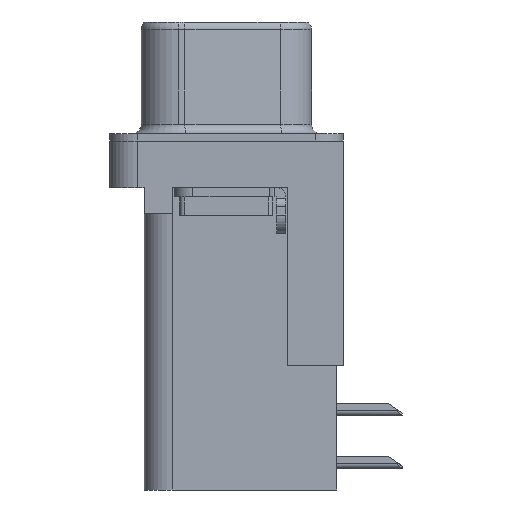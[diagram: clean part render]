
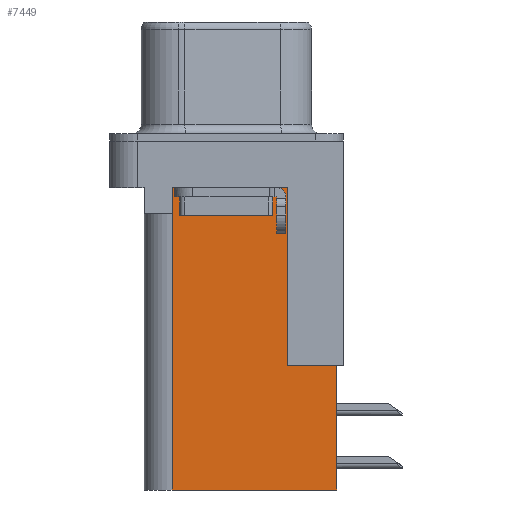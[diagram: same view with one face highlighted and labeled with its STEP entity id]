
A CAD part, left-side view. The second image highlights one B-rep face of the part: STEP entity #7449.
In plain terms, the highlighted planar face has unit normal (-1, 0, 0).
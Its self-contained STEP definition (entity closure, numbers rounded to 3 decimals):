
#61 = EDGE_CURVE ( 'NONE', #4166, #10575, #13281, .T. ) ;
#116 = CARTESIAN_POINT ( 'NONE',  ( 3.79, -3.295, -18.76 ) ) ;
#497 = VECTOR ( 'NONE', #8752, 1000. ) ;
#525 = VERTEX_POINT ( 'NONE', #11522 ) ;
#604 = CARTESIAN_POINT ( 'NONE',  ( 3.79, 2.895, -3.9 ) ) ;
#1216 = ORIENTED_EDGE ( 'NONE', *, *, #10391, .T. ) ;
#1543 = VERTEX_POINT ( 'NONE', #1921 ) ;
#1921 = CARTESIAN_POINT ( 'NONE',  ( 3.79, 2.925, -18.76 ) ) ;
#1950 = ORIENTED_EDGE ( 'NONE', *, *, #4761, .T. ) ;
#2294 = VECTOR ( 'NONE', #6717, 1000. ) ;
#2402 = VECTOR ( 'NONE', #7269, 1000. ) ;
#2490 = VECTOR ( 'NONE', #4081, 1000. ) ;
#2610 = DIRECTION ( 'NONE',  ( 0., 1., 0. ) ) ;
#3317 = VERTEX_POINT ( 'NONE', #9814 ) ;
#3702 = AXIS2_PLACEMENT_3D ( 'NONE', #116, #9983, #2610 ) ;
#4001 = VECTOR ( 'NONE', #10734, 1000. ) ;
#4081 = DIRECTION ( 'NONE',  ( 0., 1., 0. ) ) ;
#4166 = VERTEX_POINT ( 'NONE', #5208 ) ;
#4231 = DIRECTION ( 'NONE',  ( 0., 1., 0. ) ) ;
#4266 = DIRECTION ( 'NONE',  ( 0., 1., 0. ) ) ;
#4658 = EDGE_CURVE ( 'NONE', #9253, #3317, #7698, .T. ) ;
#4761 = EDGE_CURVE ( 'NONE', #3317, #525, #15623, .T. ) ;
#4988 = VERTEX_POINT ( 'NONE', #10867 ) ;
#5208 = CARTESIAN_POINT ( 'NONE',  ( 3.79, -5.925, -12.05 ) ) ;
#5492 = CARTESIAN_POINT ( 'NONE',  ( 3.79, 2.895, -3.9 ) ) ;
#6335 = ORIENTED_EDGE ( 'NONE', *, *, #7844, .T. ) ;
#6582 = VECTOR ( 'NONE', #4266, 1000. ) ;
#6639 = FACE_OUTER_BOUND ( 'NONE', #8283, .T. ) ;
#6717 = DIRECTION ( 'NONE',  ( 0., 0., 1. ) ) ;
#7216 = LINE ( 'NONE', #7931, #9690 ) ;
#7269 = DIRECTION ( 'NONE',  ( 0., 1., 0. ) ) ;
#7449 = ADVANCED_FACE ( 'NONE', ( #6639 ), #8734, .F. ) ;
#7698 = LINE ( 'NONE', #10956, #4001 ) ;
#7844 = EDGE_CURVE ( 'NONE', #12771, #4988, #8922, .T. ) ;
#7931 = CARTESIAN_POINT ( 'NONE',  ( 3.79, -6.295, -12.05 ) ) ;
#8283 = EDGE_LOOP ( 'NONE', ( #1950, #1216, #6335, #9235, #13030, #12469, #13740, #14829 ) ) ;
#8734 = PLANE ( 'NONE',  #3702 ) ;
#8752 = DIRECTION ( 'NONE',  ( 0., 0., -1. ) ) ;
#8922 = LINE ( 'NONE', #15890, #2402 ) ;
#9179 = CARTESIAN_POINT ( 'NONE',  ( 3.79, 2.925, -18.76 ) ) ;
#9183 = CARTESIAN_POINT ( 'NONE',  ( 3.79, -3.295, -18.76 ) ) ;
#9235 = ORIENTED_EDGE ( 'NONE', *, *, #12178, .F. ) ;
#9253 = VERTEX_POINT ( 'NONE', #12428 ) ;
#9469 = LINE ( 'NONE', #604, #12756 ) ;
#9690 = VECTOR ( 'NONE', #4231, 1000. ) ;
#9814 = CARTESIAN_POINT ( 'NONE',  ( 3.79, -3.295, -2.5 ) ) ;
#9853 = LINE ( 'NONE', #9183, #6582 ) ;
#9983 = DIRECTION ( 'NONE',  ( 1., 0., 0. ) ) ;
#10366 = EDGE_CURVE ( 'NONE', #10575, #1543, #9853, .T. ) ;
#10391 = EDGE_CURVE ( 'NONE', #525, #12771, #9469, .T. ) ;
#10575 = VERTEX_POINT ( 'NONE', #10910 ) ;
#10734 = DIRECTION ( 'NONE',  ( 0., 0., 1. ) ) ;
#10847 = CARTESIAN_POINT ( 'NONE',  ( 3.79, -3.295, -2.5 ) ) ;
#10867 = CARTESIAN_POINT ( 'NONE',  ( 3.79, 2.925, -3.9 ) ) ;
#10910 = CARTESIAN_POINT ( 'NONE',  ( 3.79, -5.925, -18.76 ) ) ;
#10956 = CARTESIAN_POINT ( 'NONE',  ( 3.79, -3.295, -18.76 ) ) ;
#11522 = CARTESIAN_POINT ( 'NONE',  ( 3.79, 2.895, -2.5 ) ) ;
#12178 = EDGE_CURVE ( 'NONE', #1543, #4988, #15422, .T. ) ;
#12428 = CARTESIAN_POINT ( 'NONE',  ( 3.79, -3.295, -12.05 ) ) ;
#12469 = ORIENTED_EDGE ( 'NONE', *, *, #61, .F. ) ;
#12756 = VECTOR ( 'NONE', #12924, 1000. ) ;
#12771 = VERTEX_POINT ( 'NONE', #5492 ) ;
#12924 = DIRECTION ( 'NONE',  ( 0., 0., -1. ) ) ;
#13030 = ORIENTED_EDGE ( 'NONE', *, *, #10366, .F. ) ;
#13281 = LINE ( 'NONE', #13758, #497 ) ;
#13740 = ORIENTED_EDGE ( 'NONE', *, *, #16022, .T. ) ;
#13758 = CARTESIAN_POINT ( 'NONE',  ( 3.79, -5.925, -2. ) ) ;
#14829 = ORIENTED_EDGE ( 'NONE', *, *, #4658, .T. ) ;
#15422 = LINE ( 'NONE', #9179, #2294 ) ;
#15623 = LINE ( 'NONE', #10847, #2490 ) ;
#15890 = CARTESIAN_POINT ( 'NONE',  ( 3.79, 0., -3.9 ) ) ;
#16022 = EDGE_CURVE ( 'NONE', #4166, #9253, #7216, .T. ) ;
